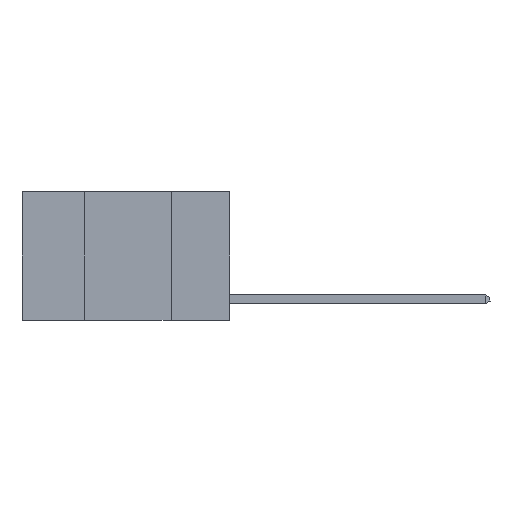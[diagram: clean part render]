
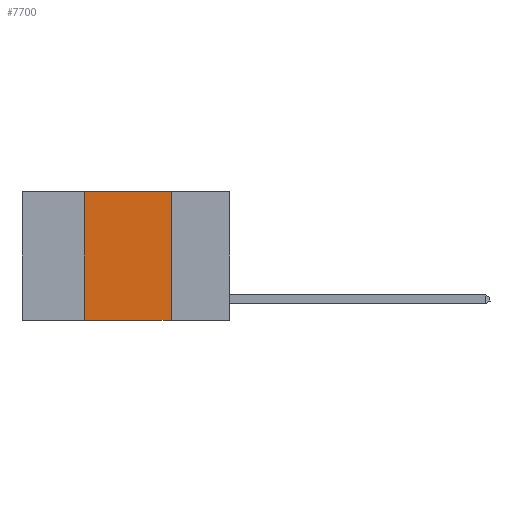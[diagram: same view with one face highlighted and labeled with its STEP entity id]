
A CAD part, left-side view. The second image highlights one B-rep face of the part: STEP entity #7700.
In plain terms, the highlighted planar face has unit normal (-1, 0, 0).
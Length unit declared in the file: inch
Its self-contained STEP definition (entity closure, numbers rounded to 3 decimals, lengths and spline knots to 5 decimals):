
#722 = ORIENTED_EDGE ( 'NONE', *, *, #2273, .F. ) ;
#2273 = EDGE_CURVE ( 'NONE', #16268, #18531, #11585, .T. ) ;
#2450 = EDGE_CURVE ( 'NONE', #6918, #19301, #22512, .T. ) ;
#3775 = FACE_OUTER_BOUND ( 'NONE', #19640, .T. ) ;
#6479 = VECTOR ( 'NONE', #17037, 39.37008 ) ;
#6730 = DIRECTION ( 'NONE',  ( 0., -1., 0. ) ) ;
#6918 = VERTEX_POINT ( 'NONE', #9987 ) ;
#7376 = VECTOR ( 'NONE', #9753, 39.37008 ) ;
#7700 = ADVANCED_FACE ( 'NONE', ( #3775 ), #23390, .F. ) ;
#8349 = DIRECTION ( 'NONE',  ( 1., 0., 0. ) ) ;
#9318 = CARTESIAN_POINT ( 'NONE',  ( 0., 0.17, 0. ) ) ;
#9753 = DIRECTION ( 'NONE',  ( 0., 0., 1. ) ) ;
#9780 = CARTESIAN_POINT ( 'NONE',  ( 0., 0.42, 0. ) ) ;
#9987 = CARTESIAN_POINT ( 'NONE',  ( 0., 0.42, -0.37 ) ) ;
#10572 = AXIS2_PLACEMENT_3D ( 'NONE', #19756, #8349, #21620 ) ;
#11585 = LINE ( 'NONE', #17292, #6479 ) ;
#12009 = LINE ( 'NONE', #21273, #12616 ) ;
#12616 = VECTOR ( 'NONE', #13814, 39.37008 ) ;
#12633 = LINE ( 'NONE', #18172, #17703 ) ;
#13814 = DIRECTION ( 'NONE',  ( 0., -1., 0. ) ) ;
#15854 = ORIENTED_EDGE ( 'NONE', *, *, #2450, .F. ) ;
#16268 = VERTEX_POINT ( 'NONE', #9318 ) ;
#17037 = DIRECTION ( 'NONE',  ( 0., 0., -1. ) ) ;
#17292 = CARTESIAN_POINT ( 'NONE',  ( 0., 0.17, 0. ) ) ;
#17703 = VECTOR ( 'NONE', #6730, 39.37008 ) ;
#18172 = CARTESIAN_POINT ( 'NONE',  ( 0., 0.6, -0.37 ) ) ;
#18531 = VERTEX_POINT ( 'NONE', #21335 ) ;
#19301 = VERTEX_POINT ( 'NONE', #23552 ) ;
#19357 = EDGE_CURVE ( 'NONE', #6918, #18531, #12633, .T. ) ;
#19640 = EDGE_LOOP ( 'NONE', ( #722, #23868, #15854, #20072 ) ) ;
#19756 = CARTESIAN_POINT ( 'NONE',  ( 0., 0.6, 0. ) ) ;
#19823 = EDGE_CURVE ( 'NONE', #19301, #16268, #12009, .T. ) ;
#20072 = ORIENTED_EDGE ( 'NONE', *, *, #19357, .T. ) ;
#21273 = CARTESIAN_POINT ( 'NONE',  ( 0., 0.6, 0. ) ) ;
#21335 = CARTESIAN_POINT ( 'NONE',  ( 0., 0.17, -0.37 ) ) ;
#21620 = DIRECTION ( 'NONE',  ( 0., 0., -1. ) ) ;
#22512 = LINE ( 'NONE', #9780, #7376 ) ;
#23390 = PLANE ( 'NONE',  #10572 ) ;
#23552 = CARTESIAN_POINT ( 'NONE',  ( 0., 0.42, 0. ) ) ;
#23868 = ORIENTED_EDGE ( 'NONE', *, *, #19823, .F. ) ;
